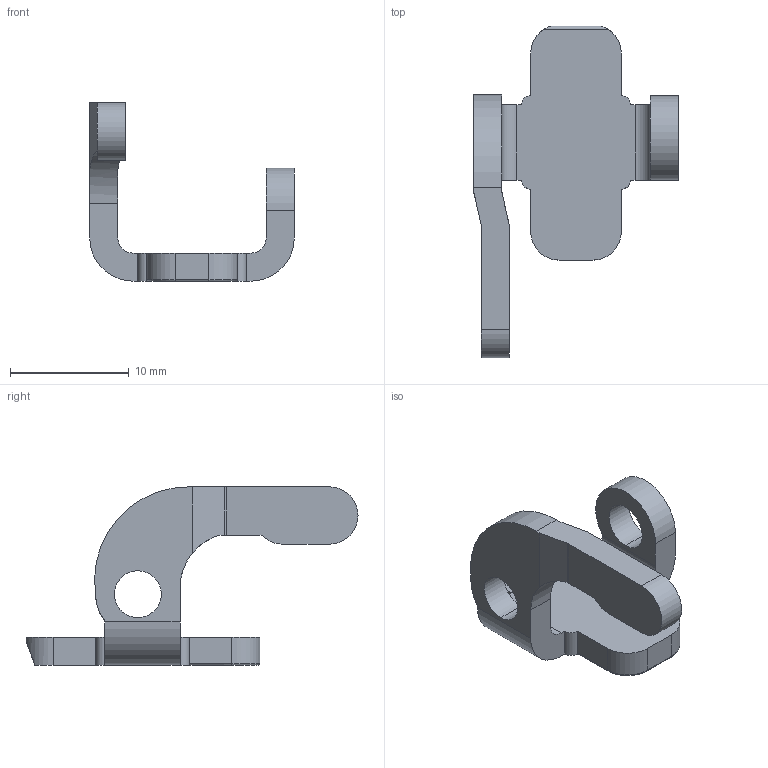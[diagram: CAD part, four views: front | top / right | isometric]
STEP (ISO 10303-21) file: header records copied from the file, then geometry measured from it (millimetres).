
FILE_DESCRIPTION((''),'2;1');
FILE_NAME('AUTO_SEAR','2019-01-20T17:52:54',('Cust'),(''),'CREO PARAMETRIC BY PTC INC, 2018300','CREO PARAMETRIC BY PTC INC, 2018300','');
FILE_SCHEMA(('AUTOMOTIVE_DESIGN { 1 0 10303 214 1 1 1 1 }'));
Length unit declared in the file: inch
Products named in the file (1): AUTO_SEAR
Bounding box: 17.22 x 27.96 x 15.01 mm (x, y, z)
Volume: 842.2 mm3; surface area: 1069.6 mm2
Topology: 1 solids, 1 shells, 56 faces, 169 edges, 115 vertices
Faces by surface type: cylinder 31, plane 23, torus 2
Entity records: 2558 total; most frequent: CARTESIAN_POINT 399, ORIENTED_EDGE 338, DIRECTION 336, PRESENTATION_STYLE_ASSIGNMENT 170, STYLED_ITEM 170, CURVE_STYLE 169, EDGE_CURVE 169, AXIS2_PLACEMENT_3D 123
